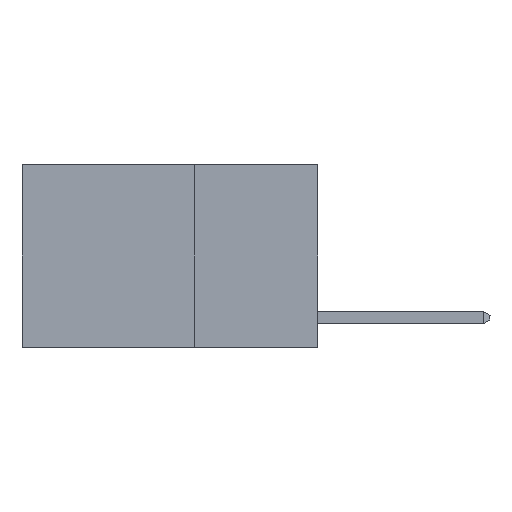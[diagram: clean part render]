
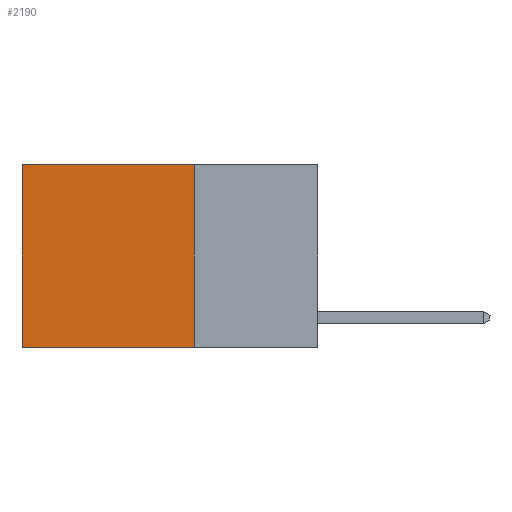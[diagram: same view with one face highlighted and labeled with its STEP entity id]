
A CAD part, left-side view. The second image highlights one B-rep face of the part: STEP entity #2190.
In plain terms, the highlighted planar face has unit normal (-1, 0, 0).
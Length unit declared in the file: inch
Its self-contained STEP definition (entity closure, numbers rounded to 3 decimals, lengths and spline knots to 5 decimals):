
#164 = VERTEX_POINT ( 'NONE', #2915 ) ;
#558 = DIRECTION ( 'NONE',  ( 0., 0., -1. ) ) ;
#1008 = LINE ( 'NONE', #5781, #2806 ) ;
#1382 = EDGE_CURVE ( 'NONE', #9417, #2944, #5410, .T. ) ;
#1437 = EDGE_LOOP ( 'NONE', ( #6289, #7330, #10264, #1877 ) ) ;
#1456 = DIRECTION ( 'NONE',  ( 0., 0., -1. ) ) ;
#1845 = EDGE_CURVE ( 'NONE', #9052, #164, #4592, .T. ) ;
#1877 = ORIENTED_EDGE ( 'NONE', *, *, #9678, .T. ) ;
#2120 = DIRECTION ( 'NONE',  ( 0., 0., -1. ) ) ;
#2190 = ADVANCED_FACE ( 'NONE', ( #6266 ), #6210, .F. ) ;
#2806 = VECTOR ( 'NONE', #6619, 39.37008 ) ;
#2915 = CARTESIAN_POINT ( 'NONE',  ( 0.2625, 0.6, -0.37 ) ) ;
#2944 = VERTEX_POINT ( 'NONE', #8253 ) ;
#2989 = CARTESIAN_POINT ( 'NONE',  ( 0.2625, 0.25, 0. ) ) ;
#2995 = CARTESIAN_POINT ( 'NONE',  ( 0.2625, 0.25, -0.37 ) ) ;
#3201 = VECTOR ( 'NONE', #1456, 39.37008 ) ;
#4072 = EDGE_CURVE ( 'NONE', #2944, #164, #6370, .T. ) ;
#4209 = VECTOR ( 'NONE', #558, 39.37008 ) ;
#4592 = LINE ( 'NONE', #6130, #4209 ) ;
#4627 = CARTESIAN_POINT ( 'NONE',  ( 0.2625, 0.25, 0. ) ) ;
#5410 = LINE ( 'NONE', #6965, #3201 ) ;
#5781 = CARTESIAN_POINT ( 'NONE',  ( 0.2625, 0.25, 0. ) ) ;
#6130 = CARTESIAN_POINT ( 'NONE',  ( 0.2625, 0.6, 0. ) ) ;
#6210 = PLANE ( 'NONE',  #9897 ) ;
#6266 = FACE_OUTER_BOUND ( 'NONE', #1437, .T. ) ;
#6289 = ORIENTED_EDGE ( 'NONE', *, *, #1845, .T. ) ;
#6370 = LINE ( 'NONE', #2995, #10072 ) ;
#6484 = CARTESIAN_POINT ( 'NONE',  ( 0.2625, 0.6, 0. ) ) ;
#6619 = DIRECTION ( 'NONE',  ( 0., 1., 0. ) ) ;
#6965 = CARTESIAN_POINT ( 'NONE',  ( 0.2625, 0.25, 0. ) ) ;
#7330 = ORIENTED_EDGE ( 'NONE', *, *, #4072, .F. ) ;
#8253 = CARTESIAN_POINT ( 'NONE',  ( 0.2625, 0.25, -0.37 ) ) ;
#9052 = VERTEX_POINT ( 'NONE', #6484 ) ;
#9417 = VERTEX_POINT ( 'NONE', #2989 ) ;
#9532 = DIRECTION ( 'NONE',  ( 0., 1., 0. ) ) ;
#9678 = EDGE_CURVE ( 'NONE', #9417, #9052, #1008, .T. ) ;
#9897 = AXIS2_PLACEMENT_3D ( 'NONE', #4627, #10187, #2120 ) ;
#10072 = VECTOR ( 'NONE', #9532, 39.37008 ) ;
#10187 = DIRECTION ( 'NONE',  ( 1., 0., 0. ) ) ;
#10264 = ORIENTED_EDGE ( 'NONE', *, *, #1382, .F. ) ;
